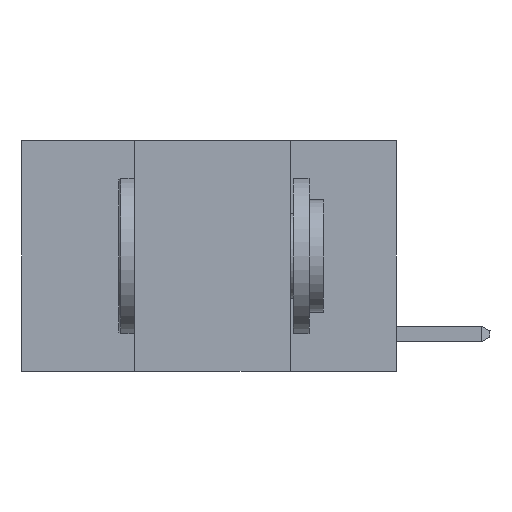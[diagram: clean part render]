
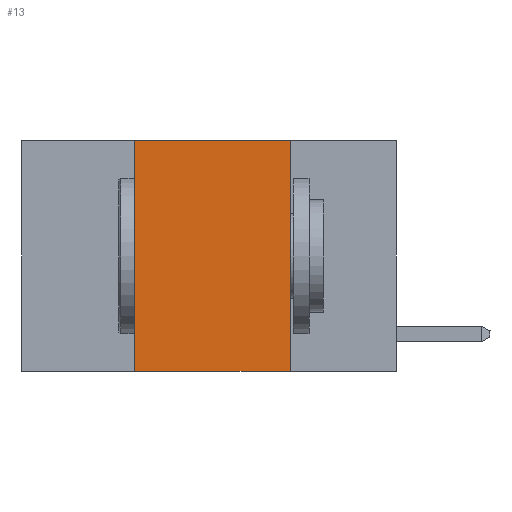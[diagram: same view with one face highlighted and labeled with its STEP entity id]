
A CAD part, left-side view. The second image highlights one B-rep face of the part: STEP entity #13.
In plain terms, the highlighted planar face has unit normal (-1, 0, 0).
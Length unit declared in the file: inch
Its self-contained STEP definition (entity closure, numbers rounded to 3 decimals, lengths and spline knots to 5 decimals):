
#13 = ADVANCED_FACE ( 'NONE', ( #14241 ), #22261, .F. ) ;
#418 = DIRECTION ( 'NONE',  ( 0., -1., 0. ) ) ;
#1623 = DIRECTION ( 'NONE',  ( 0., 0., -1. ) ) ;
#2446 = LINE ( 'NONE', #18725, #12879 ) ;
#2569 = ORIENTED_EDGE ( 'NONE', *, *, #29096, .T. ) ;
#3764 = DIRECTION ( 'NONE',  ( 1., 0., 0. ) ) ;
#5895 = DIRECTION ( 'NONE',  ( 0., 0., -1. ) ) ;
#5916 = LINE ( 'NONE', #19792, #8059 ) ;
#5932 = CARTESIAN_POINT ( 'NONE',  ( 0., 0.6, -0.37 ) ) ;
#6172 = DIRECTION ( 'NONE',  ( 0., 0., 1. ) ) ;
#6245 = VERTEX_POINT ( 'NONE', #16000 ) ;
#6584 = EDGE_CURVE ( 'NONE', #8806, #12836, #2446, .T. ) ;
#7472 = EDGE_LOOP ( 'NONE', ( #12299, #28611, #17310, #2569 ) ) ;
#8059 = VECTOR ( 'NONE', #5895, 39.37008 ) ;
#8147 = EDGE_CURVE ( 'NONE', #12836, #6245, #5916, .T. ) ;
#8806 = VERTEX_POINT ( 'NONE', #16149 ) ;
#10571 = CARTESIAN_POINT ( 'NONE',  ( 0., 0.42, 0. ) ) ;
#11707 = VECTOR ( 'NONE', #20122, 39.37008 ) ;
#12299 = ORIENTED_EDGE ( 'NONE', *, *, #8147, .F. ) ;
#12836 = VERTEX_POINT ( 'NONE', #14529 ) ;
#12878 = CARTESIAN_POINT ( 'NONE',  ( 0., 0.6, 0. ) ) ;
#12879 = VECTOR ( 'NONE', #418, 39.37008 ) ;
#14241 = FACE_OUTER_BOUND ( 'NONE', #7472, .T. ) ;
#14529 = CARTESIAN_POINT ( 'NONE',  ( 0., 0.17, 0. ) ) ;
#14906 = LINE ( 'NONE', #10571, #16706 ) ;
#16000 = CARTESIAN_POINT ( 'NONE',  ( 0., 0.17, -0.37 ) ) ;
#16149 = CARTESIAN_POINT ( 'NONE',  ( 0., 0.42, 0. ) ) ;
#16270 = VERTEX_POINT ( 'NONE', #20185 ) ;
#16706 = VECTOR ( 'NONE', #6172, 39.37008 ) ;
#17310 = ORIENTED_EDGE ( 'NONE', *, *, #22132, .F. ) ;
#18725 = CARTESIAN_POINT ( 'NONE',  ( 0., 0.6, 0. ) ) ;
#19307 = LINE ( 'NONE', #5932, #11707 ) ;
#19792 = CARTESIAN_POINT ( 'NONE',  ( 0., 0.17, 0. ) ) ;
#20122 = DIRECTION ( 'NONE',  ( 0., -1., 0. ) ) ;
#20185 = CARTESIAN_POINT ( 'NONE',  ( 0., 0.42, -0.37 ) ) ;
#22132 = EDGE_CURVE ( 'NONE', #16270, #8806, #14906, .T. ) ;
#22261 = PLANE ( 'NONE',  #27865 ) ;
#27865 = AXIS2_PLACEMENT_3D ( 'NONE', #12878, #3764, #1623 ) ;
#28611 = ORIENTED_EDGE ( 'NONE', *, *, #6584, .F. ) ;
#29096 = EDGE_CURVE ( 'NONE', #16270, #6245, #19307, .T. ) ;
